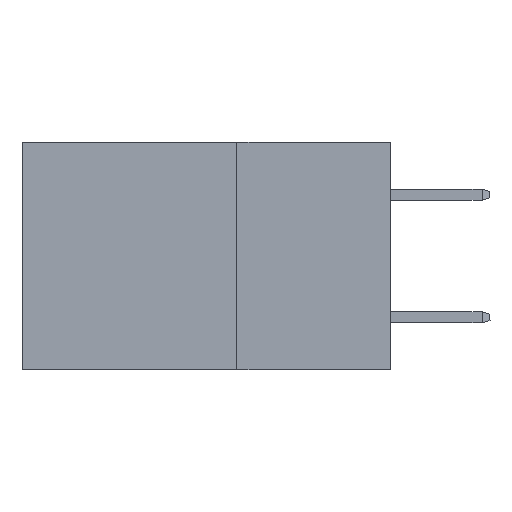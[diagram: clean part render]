
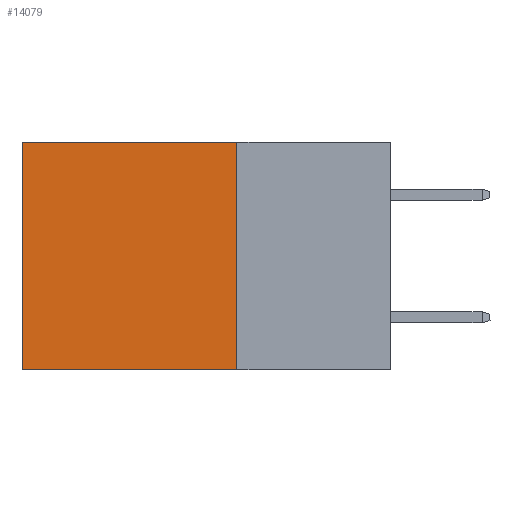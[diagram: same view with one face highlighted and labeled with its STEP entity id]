
A CAD part, left-side view. The second image highlights one B-rep face of the part: STEP entity #14079.
In plain terms, the highlighted planar face has unit normal (-1, 0, 0).
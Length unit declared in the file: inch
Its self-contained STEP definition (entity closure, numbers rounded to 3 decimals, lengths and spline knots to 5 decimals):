
#149 = VECTOR ( 'NONE', #10693, 39.37008 ) ;
#221 = CARTESIAN_POINT ( 'NONE',  ( 0.2875, 0.25, 0. ) ) ;
#284 = CARTESIAN_POINT ( 'NONE',  ( 0.2875, 0.6, -0.37 ) ) ;
#425 = CARTESIAN_POINT ( 'NONE',  ( 0.2875, 0.25, 0. ) ) ;
#664 = ORIENTED_EDGE ( 'NONE', *, *, #8940, .T. ) ;
#1060 = EDGE_CURVE ( 'NONE', #14386, #15510, #4100, .T. ) ;
#1300 = AXIS2_PLACEMENT_3D ( 'NONE', #425, #9106, #1682 ) ;
#1631 = DIRECTION ( 'NONE',  ( 0., 0., -1. ) ) ;
#1682 = DIRECTION ( 'NONE',  ( 0., 0., -1. ) ) ;
#1739 = DIRECTION ( 'NONE',  ( 0., 1., 0. ) ) ;
#2127 = VERTEX_POINT ( 'NONE', #221 ) ;
#2679 = FACE_OUTER_BOUND ( 'NONE', #14229, .T. ) ;
#2827 = ORIENTED_EDGE ( 'NONE', *, *, #12926, .F. ) ;
#3523 = LINE ( 'NONE', #6874, #149 ) ;
#3868 = EDGE_CURVE ( 'NONE', #2127, #7100, #10040, .T. ) ;
#4100 = LINE ( 'NONE', #9449, #11740 ) ;
#4395 = ORIENTED_EDGE ( 'NONE', *, *, #3868, .T. ) ;
#5640 = CARTESIAN_POINT ( 'NONE',  ( 0.2875, 0.25, -0.37 ) ) ;
#6874 = CARTESIAN_POINT ( 'NONE',  ( 0.2875, 0.25, 0. ) ) ;
#7100 = VERTEX_POINT ( 'NONE', #12591 ) ;
#8940 = EDGE_CURVE ( 'NONE', #7100, #15510, #15318, .T. ) ;
#9106 = DIRECTION ( 'NONE',  ( 1., 0., 0. ) ) ;
#9449 = CARTESIAN_POINT ( 'NONE',  ( 0.2875, 0.25, -0.37 ) ) ;
#10040 = LINE ( 'NONE', #10539, #15273 ) ;
#10539 = CARTESIAN_POINT ( 'NONE',  ( 0.2875, 0.25, 0. ) ) ;
#10693 = DIRECTION ( 'NONE',  ( 0., 0., -1. ) ) ;
#11146 = ORIENTED_EDGE ( 'NONE', *, *, #1060, .F. ) ;
#11456 = VECTOR ( 'NONE', #1631, 39.37008 ) ;
#11740 = VECTOR ( 'NONE', #1739, 39.37008 ) ;
#12591 = CARTESIAN_POINT ( 'NONE',  ( 0.2875, 0.6, 0. ) ) ;
#12926 = EDGE_CURVE ( 'NONE', #2127, #14386, #3523, .T. ) ;
#14063 = CARTESIAN_POINT ( 'NONE',  ( 0.2875, 0.6, 0. ) ) ;
#14079 = ADVANCED_FACE ( 'NONE', ( #2679 ), #14112, .F. ) ;
#14112 = PLANE ( 'NONE',  #1300 ) ;
#14229 = EDGE_LOOP ( 'NONE', ( #664, #11146, #2827, #4395 ) ) ;
#14386 = VERTEX_POINT ( 'NONE', #5640 ) ;
#15273 = VECTOR ( 'NONE', #15353, 39.37008 ) ;
#15318 = LINE ( 'NONE', #14063, #11456 ) ;
#15353 = DIRECTION ( 'NONE',  ( 0., 1., 0. ) ) ;
#15510 = VERTEX_POINT ( 'NONE', #284 ) ;
